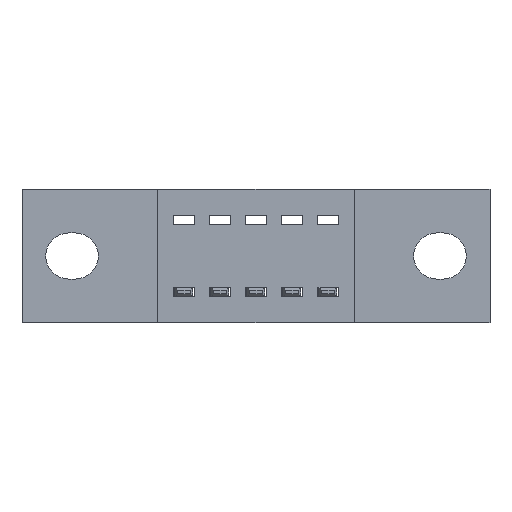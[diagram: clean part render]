
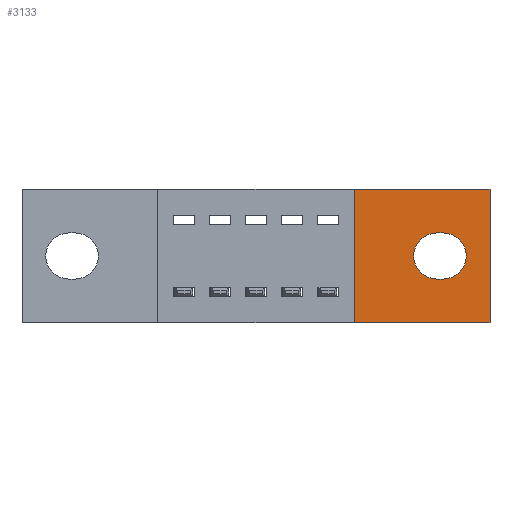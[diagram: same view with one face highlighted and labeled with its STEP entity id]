
A CAD part, front view. The second image highlights one B-rep face of the part: STEP entity #3133.
In plain terms, the highlighted planar face has unit normal (0, -1, 0).
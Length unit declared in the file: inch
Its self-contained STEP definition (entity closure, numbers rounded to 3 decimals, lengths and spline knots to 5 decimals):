
#23 = FACE_BOUND ( 'NONE', #3588, .T. ) ;
#28 = VERTEX_POINT ( 'NONE', #3714 ) ;
#126 = LINE ( 'NONE', #6352, #7627 ) ;
#358 = CARTESIAN_POINT ( 'NONE',  ( 1.17, 0., -0.249 ) ) ;
#657 = CARTESIAN_POINT ( 'NONE',  ( 1.17, 0., -0.121 ) ) ;
#746 = CARTESIAN_POINT ( 'NONE',  ( 0.923, 0., 0. ) ) ;
#748 = LINE ( 'NONE', #1607, #5074 ) ;
#797 = CIRCLE ( 'NONE', #6715, 0.064 ) ;
#1133 = ORIENTED_EDGE ( 'NONE', *, *, #2665, .F. ) ;
#1296 = EDGE_CURVE ( 'NONE', #1399, #3997, #748, .T. ) ;
#1317 = ORIENTED_EDGE ( 'NONE', *, *, #6986, .F. ) ;
#1322 = AXIS2_PLACEMENT_3D ( 'NONE', #6993, #7347, #7390 ) ;
#1399 = VERTEX_POINT ( 'NONE', #3881 ) ;
#1411 = CARTESIAN_POINT ( 'NONE',  ( 0., 0., 0. ) ) ;
#1412 = DIRECTION ( 'NONE',  ( -1., 0., 0. ) ) ;
#1607 = CARTESIAN_POINT ( 'NONE',  ( 0., 0., -0.37 ) ) ;
#1614 = FACE_OUTER_BOUND ( 'NONE', #6382, .T. ) ;
#1862 = CARTESIAN_POINT ( 'NONE',  ( 1.17, 0., -0.249 ) ) ;
#1961 = VERTEX_POINT ( 'NONE', #5753 ) ;
#2067 = VECTOR ( 'NONE', #5576, 39.37008 ) ;
#2350 = EDGE_CURVE ( 'NONE', #28, #5872, #5377, .T. ) ;
#2665 = EDGE_CURVE ( 'NONE', #4255, #6745, #4756, .T. ) ;
#2869 = EDGE_CURVE ( 'NONE', #3997, #4255, #126, .T. ) ;
#3014 = VECTOR ( 'NONE', #5119, 39.37008 ) ;
#3073 = ORIENTED_EDGE ( 'NONE', *, *, #2350, .T. ) ;
#3082 = CIRCLE ( 'NONE', #3123, 0.064 ) ;
#3123 = AXIS2_PLACEMENT_3D ( 'NONE', #3592, #3594, #4326 ) ;
#3133 = ADVANCED_FACE ( 'NONE', ( #23, #1614 ), #7105, .T. ) ;
#3160 = ORIENTED_EDGE ( 'NONE', *, *, #3788, .T. ) ;
#3195 = DIRECTION ( 'NONE',  ( 0., 0., -1. ) ) ;
#3588 = EDGE_LOOP ( 'NONE', ( #3160, #4283, #5245, #3073 ) ) ;
#3592 = CARTESIAN_POINT ( 'NONE',  ( 1.17, 0., -0.185 ) ) ;
#3594 = DIRECTION ( 'NONE',  ( 0., 1., 0. ) ) ;
#3714 = CARTESIAN_POINT ( 'NONE',  ( 1.152, 0., -0.121 ) ) ;
#3788 = EDGE_CURVE ( 'NONE', #5872, #3834, #3082, .T. ) ;
#3834 = VERTEX_POINT ( 'NONE', #1862 ) ;
#3862 = VECTOR ( 'NONE', #7355, 39.37008 ) ;
#3881 = CARTESIAN_POINT ( 'NONE',  ( 1.3, 0., -0.37 ) ) ;
#3891 = DIRECTION ( 'NONE',  ( 0., 0., -1. ) ) ;
#3997 = VERTEX_POINT ( 'NONE', #6857 ) ;
#4023 = DIRECTION ( 'NONE',  ( 0., 1., 0. ) ) ;
#4048 = CARTESIAN_POINT ( 'NONE',  ( 1.152, 0., -0.185 ) ) ;
#4255 = VERTEX_POINT ( 'NONE', #746 ) ;
#4283 = ORIENTED_EDGE ( 'NONE', *, *, #7100, .T. ) ;
#4304 = ORIENTED_EDGE ( 'NONE', *, *, #1296, .F. ) ;
#4326 = DIRECTION ( 'NONE',  ( 0., 0., -1. ) ) ;
#4335 = CARTESIAN_POINT ( 'NONE',  ( 1.3, 0., 0. ) ) ;
#4373 = VECTOR ( 'NONE', #3195, 39.37008 ) ;
#4756 = LINE ( 'NONE', #1411, #3014 ) ;
#5074 = VECTOR ( 'NONE', #1412, 39.37008 ) ;
#5075 = ORIENTED_EDGE ( 'NONE', *, *, #2869, .F. ) ;
#5119 = DIRECTION ( 'NONE',  ( 1., 0., 0. ) ) ;
#5174 = LINE ( 'NONE', #358, #2067 ) ;
#5245 = ORIENTED_EDGE ( 'NONE', *, *, #5461, .T. ) ;
#5377 = LINE ( 'NONE', #7118, #3862 ) ;
#5461 = EDGE_CURVE ( 'NONE', #1961, #28, #797, .T. ) ;
#5547 = CARTESIAN_POINT ( 'NONE',  ( 1.3, 0., 0. ) ) ;
#5576 = DIRECTION ( 'NONE',  ( -1., 0., 0. ) ) ;
#5753 = CARTESIAN_POINT ( 'NONE',  ( 1.152, 0., -0.249 ) ) ;
#5872 = VERTEX_POINT ( 'NONE', #657 ) ;
#6030 = DIRECTION ( 'NONE',  ( 0., 0., 1. ) ) ;
#6352 = CARTESIAN_POINT ( 'NONE',  ( 0.923, 0., -0.37 ) ) ;
#6382 = EDGE_LOOP ( 'NONE', ( #5075, #4304, #1317, #1133 ) ) ;
#6715 = AXIS2_PLACEMENT_3D ( 'NONE', #4048, #4023, #3891 ) ;
#6745 = VERTEX_POINT ( 'NONE', #5547 ) ;
#6857 = CARTESIAN_POINT ( 'NONE',  ( 0.923, 0., -0.37 ) ) ;
#6986 = EDGE_CURVE ( 'NONE', #6745, #1399, #7521, .T. ) ;
#6993 = CARTESIAN_POINT ( 'NONE',  ( 0., 0., -0.37 ) ) ;
#7100 = EDGE_CURVE ( 'NONE', #3834, #1961, #5174, .T. ) ;
#7105 = PLANE ( 'NONE',  #1322 ) ;
#7118 = CARTESIAN_POINT ( 'NONE',  ( 1.17, 0., -0.121 ) ) ;
#7347 = DIRECTION ( 'NONE',  ( 0., -1., 0. ) ) ;
#7355 = DIRECTION ( 'NONE',  ( 1., 0., 0. ) ) ;
#7390 = DIRECTION ( 'NONE',  ( 0., 0., -1. ) ) ;
#7521 = LINE ( 'NONE', #4335, #4373 ) ;
#7627 = VECTOR ( 'NONE', #6030, 39.37008 ) ;
